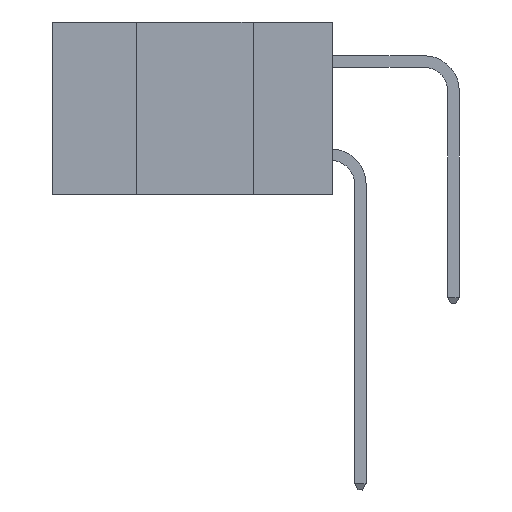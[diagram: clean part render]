
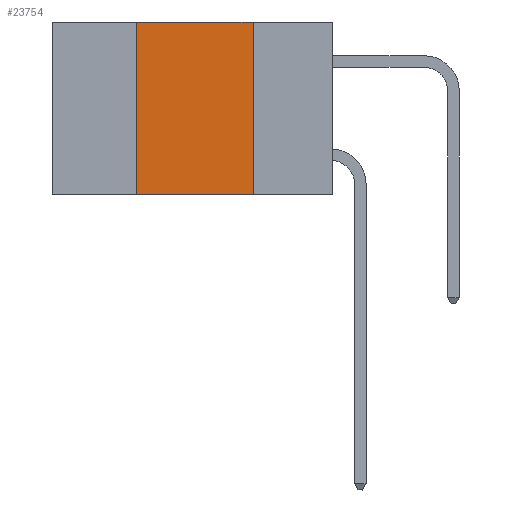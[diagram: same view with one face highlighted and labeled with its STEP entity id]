
A CAD part, left-side view. The second image highlights one B-rep face of the part: STEP entity #23754.
In plain terms, the highlighted planar face has unit normal (-1, 0, 0).
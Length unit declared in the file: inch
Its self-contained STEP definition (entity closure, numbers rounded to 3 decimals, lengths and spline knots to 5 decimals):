
#236 = ORIENTED_EDGE ( 'NONE', *, *, #22525, .F. ) ;
#316 = CARTESIAN_POINT ( 'NONE',  ( 0., 0.17, -0.37 ) ) ;
#2264 = DIRECTION ( 'NONE',  ( 0., 0., -1. ) ) ;
#2459 = CARTESIAN_POINT ( 'NONE',  ( 0., 0.6, 0. ) ) ;
#2780 = CARTESIAN_POINT ( 'NONE',  ( 0., 0.6, -0.37 ) ) ;
#4389 = CARTESIAN_POINT ( 'NONE',  ( 0., 0.17, 0. ) ) ;
#4536 = FACE_OUTER_BOUND ( 'NONE', #18543, .T. ) ;
#4729 = DIRECTION ( 'NONE',  ( 0., -1., 0. ) ) ;
#5188 = DIRECTION ( 'NONE',  ( 0., 0., 1. ) ) ;
#5560 = CARTESIAN_POINT ( 'NONE',  ( 0., 0.6, 0. ) ) ;
#6396 = DIRECTION ( 'NONE',  ( 0., -1., 0. ) ) ;
#7259 = VECTOR ( 'NONE', #2264, 39.37008 ) ;
#7686 = VECTOR ( 'NONE', #4729, 39.37008 ) ;
#8273 = CARTESIAN_POINT ( 'NONE',  ( 0., 0.17, -0.37 ) ) ;
#8638 = ORIENTED_EDGE ( 'NONE', *, *, #16098, .T. ) ;
#8809 = EDGE_CURVE ( 'NONE', #18388, #19540, #17726, .T. ) ;
#9122 = LINE ( 'NONE', #2459, #13401 ) ;
#9252 = VERTEX_POINT ( 'NONE', #8273 ) ;
#9348 = DIRECTION ( 'NONE',  ( 1., 0., 0. ) ) ;
#11256 = EDGE_CURVE ( 'NONE', #19540, #18330, #9122, .T. ) ;
#13401 = VECTOR ( 'NONE', #6396, 39.37008 ) ;
#13527 = VECTOR ( 'NONE', #5188, 39.37008 ) ;
#14613 = ORIENTED_EDGE ( 'NONE', *, *, #11256, .F. ) ;
#15082 = CARTESIAN_POINT ( 'NONE',  ( 0., 0.42, 0. ) ) ;
#15606 = CARTESIAN_POINT ( 'NONE',  ( 0., 0.42, -0.37 ) ) ;
#16098 = EDGE_CURVE ( 'NONE', #18388, #9252, #17351, .T. ) ;
#16222 = CARTESIAN_POINT ( 'NONE',  ( 0., 0.42, -0.37 ) ) ;
#16481 = PLANE ( 'NONE',  #22339 ) ;
#17351 = LINE ( 'NONE', #2780, #7686 ) ;
#17726 = LINE ( 'NONE', #16222, #13527 ) ;
#18330 = VERTEX_POINT ( 'NONE', #4389 ) ;
#18388 = VERTEX_POINT ( 'NONE', #15606 ) ;
#18543 = EDGE_LOOP ( 'NONE', ( #236, #14613, #22980, #8638 ) ) ;
#19540 = VERTEX_POINT ( 'NONE', #15082 ) ;
#21711 = LINE ( 'NONE', #316, #7259 ) ;
#21954 = DIRECTION ( 'NONE',  ( 0., 0., -1. ) ) ;
#22339 = AXIS2_PLACEMENT_3D ( 'NONE', #5560, #9348, #21954 ) ;
#22525 = EDGE_CURVE ( 'NONE', #18330, #9252, #21711, .T. ) ;
#22980 = ORIENTED_EDGE ( 'NONE', *, *, #8809, .F. ) ;
#23754 = ADVANCED_FACE ( 'NONE', ( #4536 ), #16481, .F. ) ;
